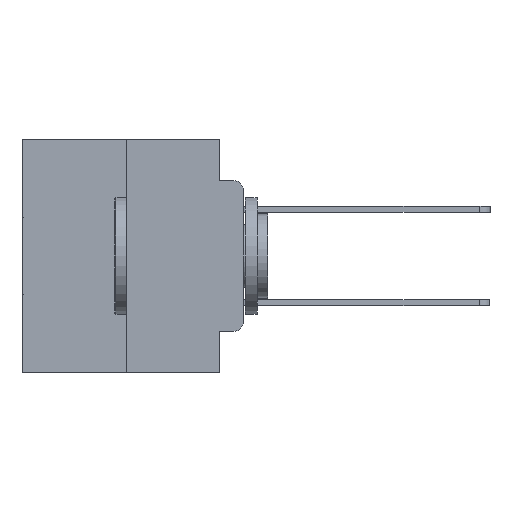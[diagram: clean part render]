
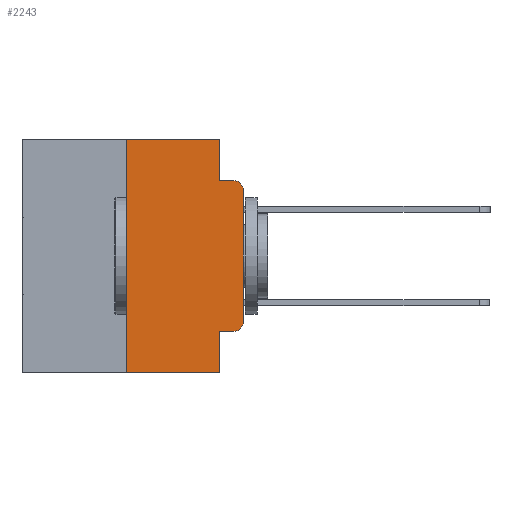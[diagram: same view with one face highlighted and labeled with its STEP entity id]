
A CAD part, left-side view. The second image highlights one B-rep face of the part: STEP entity #2243.
In plain terms, the highlighted planar face has unit normal (-1, 0, 0).
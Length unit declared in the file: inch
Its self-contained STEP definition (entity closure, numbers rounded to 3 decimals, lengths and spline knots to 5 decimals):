
#130 = AXIS2_PLACEMENT_3D ( 'NONE', #17304, #4042, #15846 ) ;
#291 = CARTESIAN_POINT ( 'NONE',  ( 0., 0.051, 0. ) ) ;
#957 = CARTESIAN_POINT ( 'NONE',  ( 0., 0.051, -0.0885 ) ) ;
#1302 = DIRECTION ( 'NONE',  ( 0., 0., 1. ) ) ;
#1589 = VERTEX_POINT ( 'NONE', #8501 ) ;
#1895 = CARTESIAN_POINT ( 'NONE',  ( 0., 0.25, -0.5 ) ) ;
#2243 = ADVANCED_FACE ( 'NONE', ( #11881 ), #4506, .F. ) ;
#2524 = AXIS2_PLACEMENT_3D ( 'NONE', #20692, #7523, #22910 ) ;
#2686 = VERTEX_POINT ( 'NONE', #17865 ) ;
#2954 = VECTOR ( 'NONE', #5674, 39.37008 ) ;
#3366 = CARTESIAN_POINT ( 'NONE',  ( 0., 0.473, 0. ) ) ;
#3888 = EDGE_CURVE ( 'NONE', #8360, #1589, #17294, .T. ) ;
#4042 = DIRECTION ( 'NONE',  ( 1., 0., 0. ) ) ;
#4441 = CARTESIAN_POINT ( 'NONE',  ( 0., 0.02, -0.3915 ) ) ;
#4506 = PLANE ( 'NONE',  #130 ) ;
#4681 = ORIENTED_EDGE ( 'NONE', *, *, #12879, .F. ) ;
#5113 = AXIS2_PLACEMENT_3D ( 'NONE', #4441, #19909, #6731 ) ;
#5674 = DIRECTION ( 'NONE',  ( 0., -1., 0. ) ) ;
#6590 = DIRECTION ( 'NONE',  ( 0., -1., 0. ) ) ;
#6731 = DIRECTION ( 'NONE',  ( 0., 0., -1. ) ) ;
#7115 = CARTESIAN_POINT ( 'NONE',  ( 0., 0.051, -0.4115 ) ) ;
#7504 = ORIENTED_EDGE ( 'NONE', *, *, #13258, .T. ) ;
#7523 = DIRECTION ( 'NONE',  ( -1., 0., 0. ) ) ;
#8360 = VERTEX_POINT ( 'NONE', #1895 ) ;
#8379 = VERTEX_POINT ( 'NONE', #17544 ) ;
#8402 = CARTESIAN_POINT ( 'NONE',  ( 0., 0.02, -0.0885 ) ) ;
#8501 = CARTESIAN_POINT ( 'NONE',  ( 0., 0.051, -0.5 ) ) ;
#9390 = ORIENTED_EDGE ( 'NONE', *, *, #19916, .F. ) ;
#9880 = CARTESIAN_POINT ( 'NONE',  ( 0., 0.051, 0. ) ) ;
#9892 = VECTOR ( 'NONE', #11546, 39.37008 ) ;
#10405 = ORIENTED_EDGE ( 'NONE', *, *, #27783, .F. ) ;
#10432 = VECTOR ( 'NONE', #12021, 39.37008 ) ;
#10525 = ORIENTED_EDGE ( 'NONE', *, *, #28481, .T. ) ;
#11407 = LINE ( 'NONE', #957, #28190 ) ;
#11546 = DIRECTION ( 'NONE',  ( 0., -1., 0. ) ) ;
#11704 = ORIENTED_EDGE ( 'NONE', *, *, #21046, .F. ) ;
#11881 = FACE_OUTER_BOUND ( 'NONE', #12756, .T. ) ;
#11890 = CARTESIAN_POINT ( 'NONE',  ( 0., 0., 0. ) ) ;
#11952 = VECTOR ( 'NONE', #1302, 39.37008 ) ;
#12021 = DIRECTION ( 'NONE',  ( 0., 0., -1. ) ) ;
#12073 = VECTOR ( 'NONE', #22666, 39.37008 ) ;
#12756 = EDGE_LOOP ( 'NONE', ( #13435, #10525, #14304, #10405, #11704, #9390, #13916, #4681, #18884, #7504 ) ) ;
#12879 = EDGE_CURVE ( 'NONE', #19222, #1589, #27890, .T. ) ;
#13089 = CARTESIAN_POINT ( 'NONE',  ( 0., 0.473, -0.5 ) ) ;
#13258 = EDGE_CURVE ( 'NONE', #2686, #8379, #24821, .T. ) ;
#13435 = ORIENTED_EDGE ( 'NONE', *, *, #27216, .T. ) ;
#13586 = EDGE_CURVE ( 'NONE', #23589, #25669, #11407, .T. ) ;
#13857 = VERTEX_POINT ( 'NONE', #24001 ) ;
#13916 = ORIENTED_EDGE ( 'NONE', *, *, #3888, .T. ) ;
#14057 = DIRECTION ( 'NONE',  ( 0., 0., 1. ) ) ;
#14304 = ORIENTED_EDGE ( 'NONE', *, *, #13586, .F. ) ;
#14365 = DIRECTION ( 'NONE',  ( 0., -1., 0. ) ) ;
#15846 = DIRECTION ( 'NONE',  ( 0., 0., -1. ) ) ;
#16592 = VECTOR ( 'NONE', #6590, 39.37008 ) ;
#16896 = CARTESIAN_POINT ( 'NONE',  ( 0., 0.25, 0. ) ) ;
#17294 = LINE ( 'NONE', #13089, #16592 ) ;
#17304 = CARTESIAN_POINT ( 'NONE',  ( 0., 0.473, 0. ) ) ;
#17544 = CARTESIAN_POINT ( 'NONE',  ( 0., 0., -0.3915 ) ) ;
#17865 = CARTESIAN_POINT ( 'NONE',  ( 0., 0.02, -0.4115 ) ) ;
#17932 = LINE ( 'NONE', #291, #12073 ) ;
#18269 = CARTESIAN_POINT ( 'NONE',  ( 0., 0.051, -0.0885 ) ) ;
#18884 = ORIENTED_EDGE ( 'NONE', *, *, #24153, .T. ) ;
#19222 = VERTEX_POINT ( 'NONE', #27966 ) ;
#19909 = DIRECTION ( 'NONE',  ( -1., 0., 0. ) ) ;
#19916 = EDGE_CURVE ( 'NONE', #8360, #27818, #23672, .T. ) ;
#20692 = CARTESIAN_POINT ( 'NONE',  ( 0., 0.02, -0.1085 ) ) ;
#21046 = EDGE_CURVE ( 'NONE', #27818, #13857, #25797, .T. ) ;
#22257 = LINE ( 'NONE', #7115, #9892 ) ;
#22261 = VERTEX_POINT ( 'NONE', #24495 ) ;
#22666 = DIRECTION ( 'NONE',  ( 0., 0., -1. ) ) ;
#22910 = DIRECTION ( 'NONE',  ( 0., 0., -1. ) ) ;
#23499 = LINE ( 'NONE', #11890, #24164 ) ;
#23589 = VERTEX_POINT ( 'NONE', #18269 ) ;
#23672 = LINE ( 'NONE', #16896, #11952 ) ;
#24001 = CARTESIAN_POINT ( 'NONE',  ( 0., 0.051, 0. ) ) ;
#24153 = EDGE_CURVE ( 'NONE', #19222, #2686, #22257, .T. ) ;
#24164 = VECTOR ( 'NONE', #14057, 39.37008 ) ;
#24495 = CARTESIAN_POINT ( 'NONE',  ( 0., 0., -0.1085 ) ) ;
#24821 = CIRCLE ( 'NONE', #5113, 0.02 ) ;
#24939 = CARTESIAN_POINT ( 'NONE',  ( 0., 0.25, 0. ) ) ;
#25669 = VERTEX_POINT ( 'NONE', #8402 ) ;
#25797 = LINE ( 'NONE', #3366, #2954 ) ;
#27216 = EDGE_CURVE ( 'NONE', #8379, #22261, #23499, .T. ) ;
#27783 = EDGE_CURVE ( 'NONE', #13857, #23589, #17932, .T. ) ;
#27802 = CIRCLE ( 'NONE', #2524, 0.02 ) ;
#27818 = VERTEX_POINT ( 'NONE', #24939 ) ;
#27890 = LINE ( 'NONE', #9880, #10432 ) ;
#27966 = CARTESIAN_POINT ( 'NONE',  ( 0., 0.051, -0.4115 ) ) ;
#28190 = VECTOR ( 'NONE', #14365, 39.37008 ) ;
#28481 = EDGE_CURVE ( 'NONE', #22261, #25669, #27802, .T. ) ;
